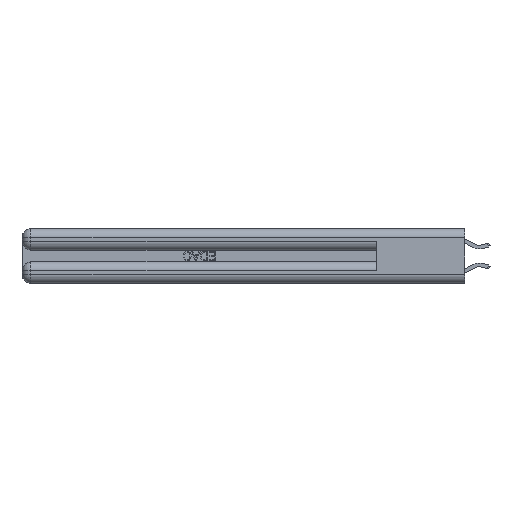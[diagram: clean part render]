
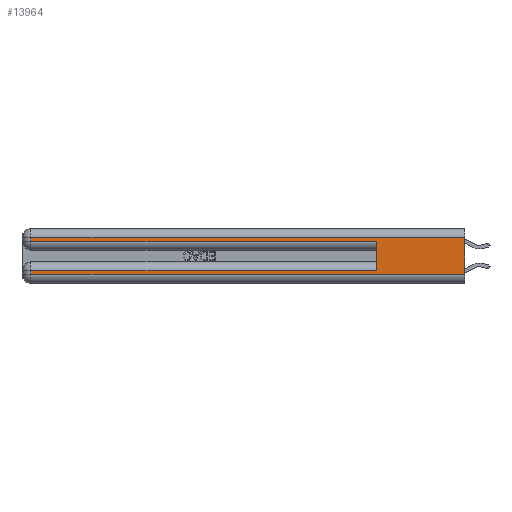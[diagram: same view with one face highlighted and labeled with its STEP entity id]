
A CAD part, left-side view. The second image highlights one B-rep face of the part: STEP entity #13964.
In plain terms, the highlighted planar face has unit normal (-1, 0, 0).
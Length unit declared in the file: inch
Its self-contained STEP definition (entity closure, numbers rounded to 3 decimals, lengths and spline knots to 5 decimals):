
#881 = AXIS2_PLACEMENT_3D ( 'NONE', #22808, #7366, #27710 ) ;
#1463 = PLANE ( 'NONE',  #881 ) ;
#1639 = VECTOR ( 'NONE', #15995, 39.37008 ) ;
#1760 = VERTEX_POINT ( 'NONE', #20705 ) ;
#2455 = DIRECTION ( 'NONE',  ( 0., -1., 0. ) ) ;
#2572 = CARTESIAN_POINT ( 'NONE',  ( 0., 0., 0.31 ) ) ;
#2676 = ORIENTED_EDGE ( 'NONE', *, *, #8669, .F. ) ;
#3163 = EDGE_CURVE ( 'NONE', #24145, #18177, #21191, .T. ) ;
#3455 = VERTEX_POINT ( 'NONE', #17700 ) ;
#3472 = LINE ( 'NONE', #19643, #14076 ) ;
#4301 = VECTOR ( 'NONE', #18381, 39.37008 ) ;
#4728 = CARTESIAN_POINT ( 'NONE',  ( 0., 2.94, 0.285 ) ) ;
#5617 = DIRECTION ( 'NONE',  ( 0., 0., -1. ) ) ;
#6802 = CARTESIAN_POINT ( 'NONE',  ( 0., 0., 0.31 ) ) ;
#7366 = DIRECTION ( 'NONE',  ( 1., 0., 0. ) ) ;
#7624 = CARTESIAN_POINT ( 'NONE',  ( 0., 0.6, 0.285 ) ) ;
#8332 = DIRECTION ( 'NONE',  ( 0., 0., 1. ) ) ;
#8669 = EDGE_CURVE ( 'NONE', #15270, #1760, #19132, .T. ) ;
#9216 = VECTOR ( 'NONE', #8332, 39.37008 ) ;
#10876 = ORIENTED_EDGE ( 'NONE', *, *, #18073, .T. ) ;
#11671 = CARTESIAN_POINT ( 'NONE',  ( 0., 2.94, 0.37 ) ) ;
#11950 = EDGE_CURVE ( 'NONE', #15270, #18892, #15943, .T. ) ;
#12374 = FACE_OUTER_BOUND ( 'NONE', #14969, .T. ) ;
#12430 = VECTOR ( 'NONE', #19487, 39.37008 ) ;
#13900 = CARTESIAN_POINT ( 'NONE',  ( 0., 0., 0.37 ) ) ;
#13964 = ADVANCED_FACE ( 'NONE', ( #12374 ), #1463, .F. ) ;
#14076 = VECTOR ( 'NONE', #17032, 39.37008 ) ;
#14969 = EDGE_LOOP ( 'NONE', ( #2676, #18973, #10876, #25246, #33790, #20838, #22280, #27192 ) ) ;
#15270 = VERTEX_POINT ( 'NONE', #6802 ) ;
#15635 = CARTESIAN_POINT ( 'NONE',  ( 0., 2.94, 0.085 ) ) ;
#15943 = LINE ( 'NONE', #2572, #4301 ) ;
#15995 = DIRECTION ( 'NONE',  ( 0., -1., 0. ) ) ;
#16148 = CARTESIAN_POINT ( 'NONE',  ( 0., 0.6, 0.145 ) ) ;
#16158 = CARTESIAN_POINT ( 'NONE',  ( 0., 0., 0.285 ) ) ;
#17032 = DIRECTION ( 'NONE',  ( 0., 0., -1. ) ) ;
#17595 = CARTESIAN_POINT ( 'NONE',  ( 0., 0., 0.085 ) ) ;
#17700 = CARTESIAN_POINT ( 'NONE',  ( 0., 2.94, 0.06 ) ) ;
#18073 = EDGE_CURVE ( 'NONE', #18892, #24145, #24699, .T. ) ;
#18177 = VERTEX_POINT ( 'NONE', #7624 ) ;
#18381 = DIRECTION ( 'NONE',  ( 0., 1., 0. ) ) ;
#18659 = VECTOR ( 'NONE', #5617, 39.37008 ) ;
#18892 = VERTEX_POINT ( 'NONE', #27359 ) ;
#18973 = ORIENTED_EDGE ( 'NONE', *, *, #11950, .T. ) ;
#19106 = EDGE_CURVE ( 'NONE', #25788, #19762, #20047, .T. ) ;
#19132 = LINE ( 'NONE', #13900, #12430 ) ;
#19142 = CARTESIAN_POINT ( 'NONE',  ( 0., 0.6, 0.085 ) ) ;
#19487 = DIRECTION ( 'NONE',  ( 0., 0., -1. ) ) ;
#19643 = CARTESIAN_POINT ( 'NONE',  ( 0., 2.94, 0.37 ) ) ;
#19762 = VERTEX_POINT ( 'NONE', #15635 ) ;
#19873 = DIRECTION ( 'NONE',  ( 0., 1., 0. ) ) ;
#19896 = EDGE_CURVE ( 'NONE', #25788, #18177, #31960, .T. ) ;
#20047 = LINE ( 'NONE', #17595, #29724 ) ;
#20705 = CARTESIAN_POINT ( 'NONE',  ( 0., 0., 0.06 ) ) ;
#20838 = ORIENTED_EDGE ( 'NONE', *, *, #19106, .T. ) ;
#21191 = LINE ( 'NONE', #16158, #1639 ) ;
#22280 = ORIENTED_EDGE ( 'NONE', *, *, #34069, .T. ) ;
#22808 = CARTESIAN_POINT ( 'NONE',  ( 0., 0., 0.37 ) ) ;
#24145 = VERTEX_POINT ( 'NONE', #4728 ) ;
#24699 = LINE ( 'NONE', #11671, #18659 ) ;
#25246 = ORIENTED_EDGE ( 'NONE', *, *, #3163, .T. ) ;
#25788 = VERTEX_POINT ( 'NONE', #19142 ) ;
#27192 = ORIENTED_EDGE ( 'NONE', *, *, #27726, .T. ) ;
#27359 = CARTESIAN_POINT ( 'NONE',  ( 0., 2.94, 0.31 ) ) ;
#27710 = DIRECTION ( 'NONE',  ( 0., 0., -1. ) ) ;
#27726 = EDGE_CURVE ( 'NONE', #3455, #1760, #29547, .T. ) ;
#29547 = LINE ( 'NONE', #34242, #31120 ) ;
#29724 = VECTOR ( 'NONE', #19873, 39.37008 ) ;
#31120 = VECTOR ( 'NONE', #2455, 39.37008 ) ;
#31960 = LINE ( 'NONE', #16148, #9216 ) ;
#33790 = ORIENTED_EDGE ( 'NONE', *, *, #19896, .F. ) ;
#34069 = EDGE_CURVE ( 'NONE', #19762, #3455, #3472, .T. ) ;
#34242 = CARTESIAN_POINT ( 'NONE',  ( 0., 0., 0.06 ) ) ;
